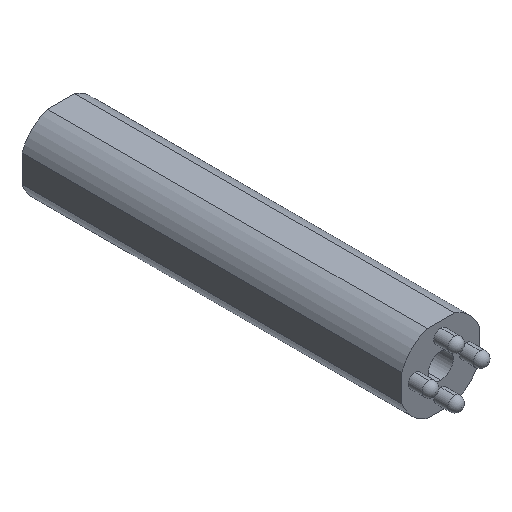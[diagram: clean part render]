
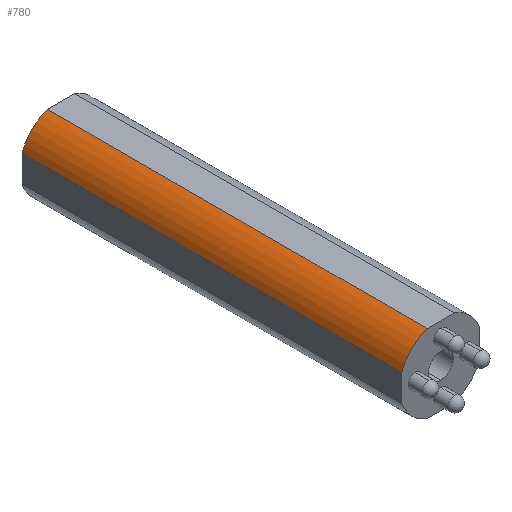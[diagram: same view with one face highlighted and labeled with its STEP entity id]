
A CAD part, isometric view. The second image highlights one B-rep face of the part: STEP entity #780.
In plain terms, the highlighted cylindrical face has radius 15.145 mm (diameter 30.29 mm), a partial arc.
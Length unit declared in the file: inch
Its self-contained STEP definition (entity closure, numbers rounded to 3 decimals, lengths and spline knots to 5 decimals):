
#4 = VERTEX_POINT ( 'NONE', #129 ) ;
#6 = VERTEX_POINT ( 'NONE', #140 ) ;
#27 = VERTEX_POINT ( 'NONE', #152 ) ;
#28 = VERTEX_POINT ( 'NONE', #137 ) ;
#42 = EDGE_LOOP ( 'NONE', ( #272, #274, #271, #257 ) ) ;
#129 = CARTESIAN_POINT ( 'NONE',  ( 0.36633, 5.5, 0.3661 ) ) ;
#137 = CARTESIAN_POINT ( 'NONE',  ( 0.36633, 0., 0.3661 ) ) ;
#140 = CARTESIAN_POINT ( 'NONE',  ( 0., 5.5, 0. ) ) ;
#152 = CARTESIAN_POINT ( 'NONE',  ( 0., 0., 0. ) ) ;
#257 = ORIENTED_EDGE ( 'NONE', *, *, #742, .T. ) ;
#271 = ORIENTED_EDGE ( 'NONE', *, *, #765, .F. ) ;
#272 = ORIENTED_EDGE ( 'NONE', *, *, #712, .T. ) ;
#274 = ORIENTED_EDGE ( 'NONE', *, *, #738, .F. ) ;
#363 = CARTESIAN_POINT ( 'NONE',  ( 0.56283, 0., -0.19685 ) ) ;
#364 = DIRECTION ( 'NONE',  ( 0., 1., 0. ) ) ;
#366 = DIRECTION ( 'NONE',  ( 0., 0., 1. ) ) ;
#456 = CARTESIAN_POINT ( 'NONE',  ( 0., 5.5, 0. ) ) ;
#463 = LINE ( 'NONE', #478, #901 ) ;
#478 = CARTESIAN_POINT ( 'NONE',  ( 0.36633, 5.5, 0.3661 ) ) ;
#482 = DIRECTION ( 'NONE',  ( 0., -1., 0. ) ) ;
#483 = LINE ( 'NONE', #456, #899 ) ;
#484 = DIRECTION ( 'NONE',  ( 0., -1., 0. ) ) ;
#540 = CARTESIAN_POINT ( 'NONE',  ( 0.56283, 5.5, -0.19685 ) ) ;
#541 = DIRECTION ( 'NONE',  ( 0., 1., 0. ) ) ;
#544 = DIRECTION ( 'NONE',  ( 0., 0., 1. ) ) ;
#596 = DIRECTION ( 'NONE',  ( 0., -1., 0. ) ) ;
#597 = DIRECTION ( 'NONE',  ( 0., 0., -1. ) ) ;
#602 = CARTESIAN_POINT ( 'NONE',  ( 0.56283, 5.5, -0.19685 ) ) ;
#712 = EDGE_CURVE ( 'NONE', #27, #28, #812, .T. ) ;
#738 = EDGE_CURVE ( 'NONE', #4, #28, #463, .T. ) ;
#742 = EDGE_CURVE ( 'NONE', #6, #27, #483, .T. ) ;
#765 = EDGE_CURVE ( 'NONE', #6, #4, #837, .T. ) ;
#780 = ADVANCED_FACE ( 'NONE', ( #967 ), #969, .T. ) ;
#812 = CIRCLE ( 'NONE', #858, 0.59626 ) ;
#837 = CIRCLE ( 'NONE', #925, 0.59626 ) ;
#858 = AXIS2_PLACEMENT_3D ( 'NONE', #363, #364, #366 ) ;
#899 = VECTOR ( 'NONE', #484, 39.37008 ) ;
#901 = VECTOR ( 'NONE', #482, 39.37008 ) ;
#925 = AXIS2_PLACEMENT_3D ( 'NONE', #540, #541, #544 ) ;
#967 = FACE_OUTER_BOUND ( 'NONE', #42, .T. ) ;
#969 = CYLINDRICAL_SURFACE ( 'NONE', #970, 0.59626 ) ;
#970 = AXIS2_PLACEMENT_3D ( 'NONE', #602, #596, #597 ) ;
